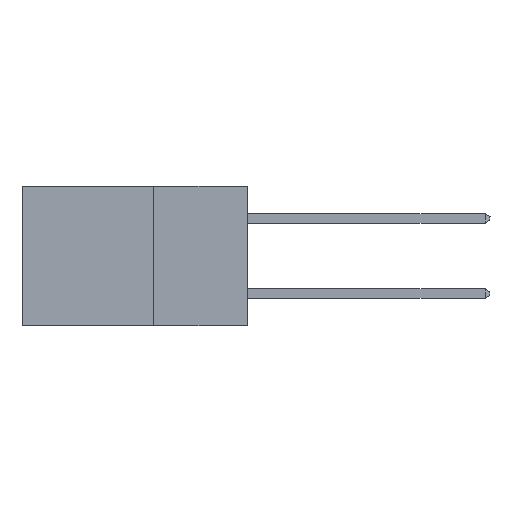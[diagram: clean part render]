
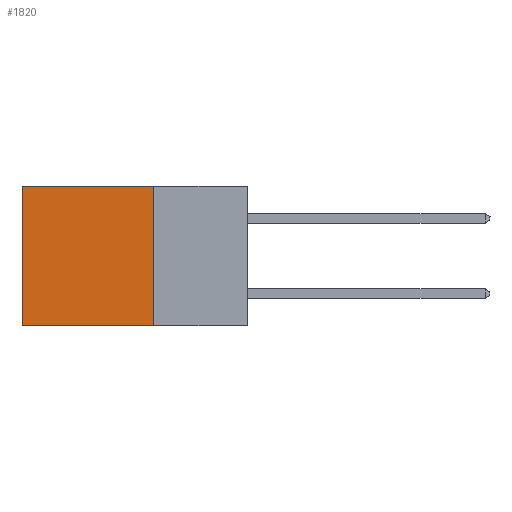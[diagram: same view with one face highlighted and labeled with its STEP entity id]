
A CAD part, left-side view. The second image highlights one B-rep face of the part: STEP entity #1820.
In plain terms, the highlighted planar face has unit normal (-1, 0, 0).
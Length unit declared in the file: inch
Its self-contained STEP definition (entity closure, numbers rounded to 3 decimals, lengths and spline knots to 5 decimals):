
#330 = CARTESIAN_POINT ( 'NONE',  ( 0.2615, 0.6, -0.37 ) ) ;
#606 = FACE_OUTER_BOUND ( 'NONE', #4689, .T. ) ;
#736 = ORIENTED_EDGE ( 'NONE', *, *, #6630, .F. ) ;
#1820 = ADVANCED_FACE ( 'NONE', ( #606 ), #15511, .F. ) ;
#1900 = VERTEX_POINT ( 'NONE', #14916 ) ;
#1980 = CARTESIAN_POINT ( 'NONE',  ( 0.2615, 0.25, -0.37 ) ) ;
#3750 = CARTESIAN_POINT ( 'NONE',  ( 0.2615, 0.6, -0.37 ) ) ;
#3976 = LINE ( 'NONE', #8987, #9745 ) ;
#4208 = CARTESIAN_POINT ( 'NONE',  ( 0.2615, 0.25, -0.37 ) ) ;
#4560 = VERTEX_POINT ( 'NONE', #14429 ) ;
#4689 = EDGE_LOOP ( 'NONE', ( #16142, #736, #11293, #7118 ) ) ;
#4785 = LINE ( 'NONE', #1980, #15218 ) ;
#5325 = DIRECTION ( 'NONE',  ( 0., 0., -1. ) ) ;
#5442 = DIRECTION ( 'NONE',  ( 0., 0., -1. ) ) ;
#6057 = VERTEX_POINT ( 'NONE', #12719 ) ;
#6555 = LINE ( 'NONE', #330, #10552 ) ;
#6621 = LINE ( 'NONE', #14215, #9309 ) ;
#6630 = EDGE_CURVE ( 'NONE', #6057, #15190, #4785, .T. ) ;
#6876 = DIRECTION ( 'NONE',  ( 0., 0., -1. ) ) ;
#7118 = ORIENTED_EDGE ( 'NONE', *, *, #11474, .T. ) ;
#7221 = AXIS2_PLACEMENT_3D ( 'NONE', #4208, #9381, #5442 ) ;
#7334 = DIRECTION ( 'NONE',  ( 0., 1., 0. ) ) ;
#7753 = DIRECTION ( 'NONE',  ( 0., 1., 0. ) ) ;
#8987 = CARTESIAN_POINT ( 'NONE',  ( 0.2615, 0.25, 0. ) ) ;
#9309 = VECTOR ( 'NONE', #6876, 39.37008 ) ;
#9381 = DIRECTION ( 'NONE',  ( 1., 0., 0. ) ) ;
#9745 = VECTOR ( 'NONE', #7753, 39.37008 ) ;
#10552 = VECTOR ( 'NONE', #5325, 39.37008 ) ;
#11293 = ORIENTED_EDGE ( 'NONE', *, *, #16093, .F. ) ;
#11474 = EDGE_CURVE ( 'NONE', #1900, #4560, #3976, .T. ) ;
#12719 = CARTESIAN_POINT ( 'NONE',  ( 0.2615, 0.25, -0.37 ) ) ;
#13079 = EDGE_CURVE ( 'NONE', #4560, #15190, #6555, .T. ) ;
#14215 = CARTESIAN_POINT ( 'NONE',  ( 0.2615, 0.25, -0.37 ) ) ;
#14429 = CARTESIAN_POINT ( 'NONE',  ( 0.2615, 0.6, 0. ) ) ;
#14916 = CARTESIAN_POINT ( 'NONE',  ( 0.2615, 0.25, 0. ) ) ;
#15190 = VERTEX_POINT ( 'NONE', #3750 ) ;
#15218 = VECTOR ( 'NONE', #7334, 39.37008 ) ;
#15511 = PLANE ( 'NONE',  #7221 ) ;
#16093 = EDGE_CURVE ( 'NONE', #1900, #6057, #6621, .T. ) ;
#16142 = ORIENTED_EDGE ( 'NONE', *, *, #13079, .T. ) ;
